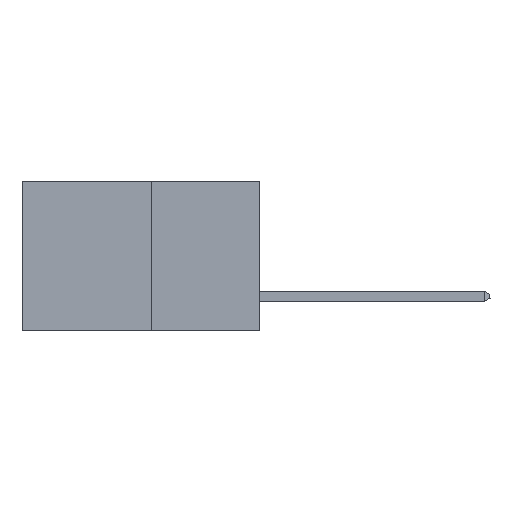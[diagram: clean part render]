
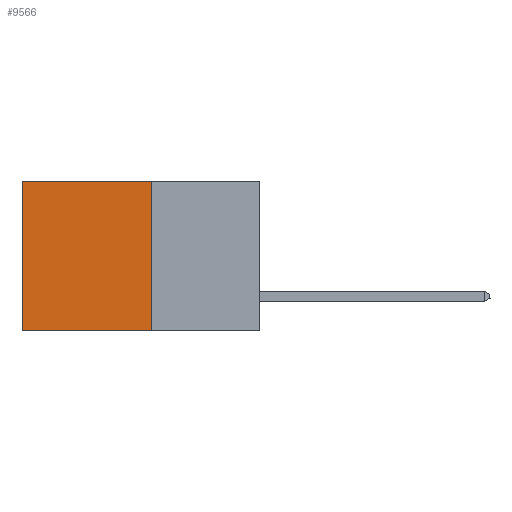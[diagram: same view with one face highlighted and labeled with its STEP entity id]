
A CAD part, left-side view. The second image highlights one B-rep face of the part: STEP entity #9566.
In plain terms, the highlighted planar face has unit normal (-1, 0, 0).
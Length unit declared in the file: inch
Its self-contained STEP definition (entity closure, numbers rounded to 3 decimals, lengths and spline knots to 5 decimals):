
#157 = LINE ( 'NONE', #7545, #7516 ) ;
#1400 = EDGE_CURVE ( 'NONE', #10176, #4868, #9953, .T. ) ;
#1838 = EDGE_CURVE ( 'NONE', #4868, #12422, #13937, .T. ) ;
#2691 = ORIENTED_EDGE ( 'NONE', *, *, #7556, .T. ) ;
#2699 = DIRECTION ( 'NONE',  ( 1., 0., 0. ) ) ;
#2909 = CARTESIAN_POINT ( 'NONE',  ( 0.277, 0.59, -0.37 ) ) ;
#3929 = FACE_OUTER_BOUND ( 'NONE', #7853, .T. ) ;
#3976 = ORIENTED_EDGE ( 'NONE', *, *, #1838, .F. ) ;
#4868 = VERTEX_POINT ( 'NONE', #7195 ) ;
#5257 = AXIS2_PLACEMENT_3D ( 'NONE', #10959, #2699, #16332 ) ;
#5742 = VECTOR ( 'NONE', #16533, 39.37008 ) ;
#7195 = CARTESIAN_POINT ( 'NONE',  ( 0.277, 0.27, -0.37 ) ) ;
#7328 = CARTESIAN_POINT ( 'NONE',  ( 0.277, 0.59, 0. ) ) ;
#7516 = VECTOR ( 'NONE', #15634, 39.37008 ) ;
#7545 = CARTESIAN_POINT ( 'NONE',  ( 0.277, 0.27, 0. ) ) ;
#7556 = EDGE_CURVE ( 'NONE', #10176, #12340, #157, .T. ) ;
#7853 = EDGE_LOOP ( 'NONE', ( #9192, #3976, #11531, #2691 ) ) ;
#8342 = EDGE_CURVE ( 'NONE', #12340, #12422, #9423, .T. ) ;
#8893 = CARTESIAN_POINT ( 'NONE',  ( 0.277, 0.59, -0.37 ) ) ;
#9192 = ORIENTED_EDGE ( 'NONE', *, *, #8342, .T. ) ;
#9423 = LINE ( 'NONE', #2909, #5742 ) ;
#9566 = ADVANCED_FACE ( 'NONE', ( #3929 ), #13676, .F. ) ;
#9936 = VECTOR ( 'NONE', #12626, 39.37008 ) ;
#9953 = LINE ( 'NONE', #10731, #13114 ) ;
#10176 = VERTEX_POINT ( 'NONE', #13536 ) ;
#10731 = CARTESIAN_POINT ( 'NONE',  ( 0.277, 0.27, -0.37 ) ) ;
#10959 = CARTESIAN_POINT ( 'NONE',  ( 0.277, 0.27, -0.37 ) ) ;
#11531 = ORIENTED_EDGE ( 'NONE', *, *, #1400, .F. ) ;
#12271 = DIRECTION ( 'NONE',  ( 0., 0., -1. ) ) ;
#12340 = VERTEX_POINT ( 'NONE', #7328 ) ;
#12422 = VERTEX_POINT ( 'NONE', #8893 ) ;
#12626 = DIRECTION ( 'NONE',  ( 0., 1., 0. ) ) ;
#13114 = VECTOR ( 'NONE', #12271, 39.37008 ) ;
#13536 = CARTESIAN_POINT ( 'NONE',  ( 0.277, 0.27, 0. ) ) ;
#13676 = PLANE ( 'NONE',  #5257 ) ;
#13937 = LINE ( 'NONE', #15721, #9936 ) ;
#15634 = DIRECTION ( 'NONE',  ( 0., 1., 0. ) ) ;
#15721 = CARTESIAN_POINT ( 'NONE',  ( 0.277, 0.27, -0.37 ) ) ;
#16332 = DIRECTION ( 'NONE',  ( 0., 0., -1. ) ) ;
#16533 = DIRECTION ( 'NONE',  ( 0., 0., -1. ) ) ;
